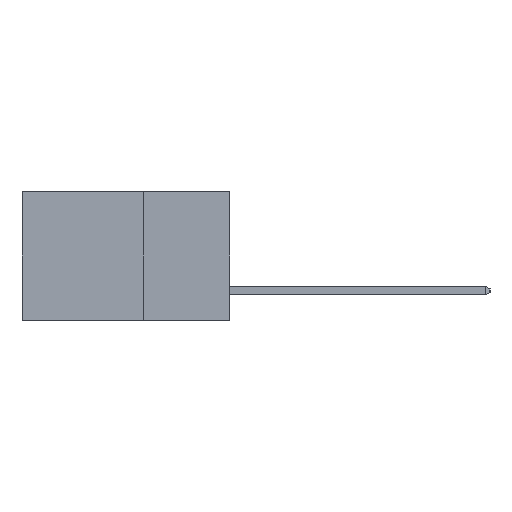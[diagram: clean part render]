
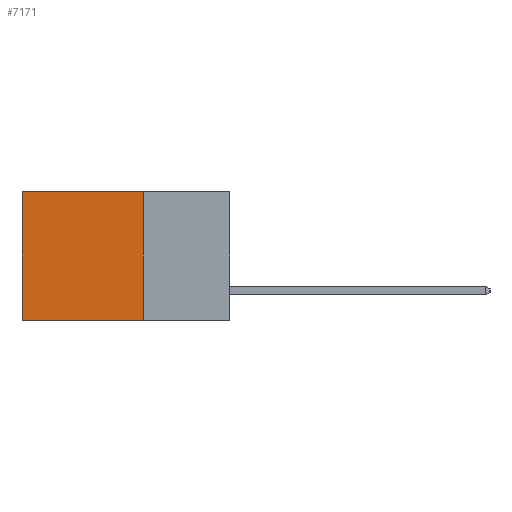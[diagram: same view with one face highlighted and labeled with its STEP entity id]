
A CAD part, left-side view. The second image highlights one B-rep face of the part: STEP entity #7171.
In plain terms, the highlighted planar face has unit normal (-1, 0, 0).
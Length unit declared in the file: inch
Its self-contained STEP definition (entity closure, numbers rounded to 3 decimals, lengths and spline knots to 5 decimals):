
#528 = ORIENTED_EDGE ( 'NONE', *, *, #11438, .T. ) ;
#563 = AXIS2_PLACEMENT_3D ( 'NONE', #10298, #10135, #10085 ) ;
#2044 = CARTESIAN_POINT ( 'NONE',  ( 0.298, 0.25, -0.37 ) ) ;
#2138 = VECTOR ( 'NONE', #12346, 39.37008 ) ;
#3075 = CARTESIAN_POINT ( 'NONE',  ( 0.298, 0.25, 0. ) ) ;
#4198 = VECTOR ( 'NONE', #7319, 39.37008 ) ;
#4338 = VERTEX_POINT ( 'NONE', #17619 ) ;
#4853 = VERTEX_POINT ( 'NONE', #20384 ) ;
#5290 = EDGE_CURVE ( 'NONE', #13785, #7297, #6515, .T. ) ;
#5698 = CARTESIAN_POINT ( 'NONE',  ( 0.298, 0.6, 0. ) ) ;
#6515 = LINE ( 'NONE', #13181, #2138 ) ;
#6766 = VECTOR ( 'NONE', #19126, 39.37008 ) ;
#7171 = ADVANCED_FACE ( 'NONE', ( #8475 ), #10620, .F. ) ;
#7297 = VERTEX_POINT ( 'NONE', #8171 ) ;
#7319 = DIRECTION ( 'NONE',  ( 0., 0., -1. ) ) ;
#7657 = ORIENTED_EDGE ( 'NONE', *, *, #19577, .F. ) ;
#7793 = LINE ( 'NONE', #15914, #6766 ) ;
#8171 = CARTESIAN_POINT ( 'NONE',  ( 0.298, 0.25, -0.37 ) ) ;
#8475 = FACE_OUTER_BOUND ( 'NONE', #15586, .T. ) ;
#9535 = VECTOR ( 'NONE', #11818, 39.37008 ) ;
#10085 = DIRECTION ( 'NONE',  ( 0., 0., -1. ) ) ;
#10135 = DIRECTION ( 'NONE',  ( 1., 0., 0. ) ) ;
#10298 = CARTESIAN_POINT ( 'NONE',  ( 0.298, 0.25, 0. ) ) ;
#10620 = PLANE ( 'NONE',  #563 ) ;
#11438 = EDGE_CURVE ( 'NONE', #4853, #4338, #12818, .T. ) ;
#11744 = EDGE_CURVE ( 'NONE', #13785, #4853, #7793, .T. ) ;
#11818 = DIRECTION ( 'NONE',  ( 0., 1., 0. ) ) ;
#12346 = DIRECTION ( 'NONE',  ( 0., 0., -1. ) ) ;
#12733 = ORIENTED_EDGE ( 'NONE', *, *, #11744, .T. ) ;
#12818 = LINE ( 'NONE', #5698, #4198 ) ;
#13181 = CARTESIAN_POINT ( 'NONE',  ( 0.298, 0.25, 0. ) ) ;
#13785 = VERTEX_POINT ( 'NONE', #3075 ) ;
#14274 = LINE ( 'NONE', #2044, #9535 ) ;
#15586 = EDGE_LOOP ( 'NONE', ( #528, #7657, #16407, #12733 ) ) ;
#15914 = CARTESIAN_POINT ( 'NONE',  ( 0.298, 0.25, 0. ) ) ;
#16407 = ORIENTED_EDGE ( 'NONE', *, *, #5290, .F. ) ;
#17619 = CARTESIAN_POINT ( 'NONE',  ( 0.298, 0.6, -0.37 ) ) ;
#19126 = DIRECTION ( 'NONE',  ( 0., 1., 0. ) ) ;
#19577 = EDGE_CURVE ( 'NONE', #7297, #4338, #14274, .T. ) ;
#20384 = CARTESIAN_POINT ( 'NONE',  ( 0.298, 0.6, 0. ) ) ;
